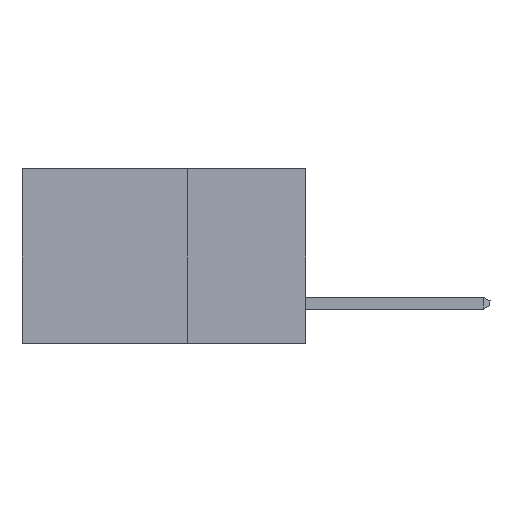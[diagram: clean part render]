
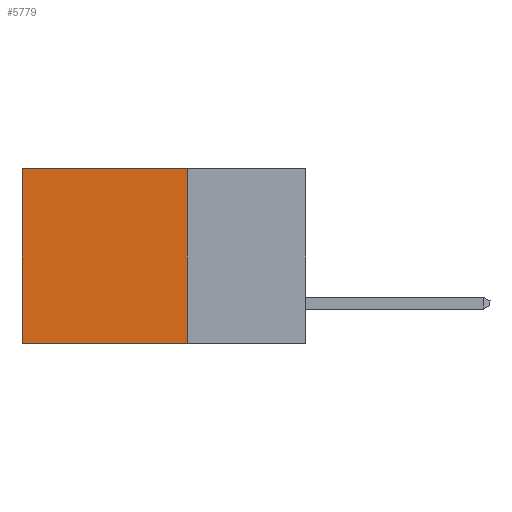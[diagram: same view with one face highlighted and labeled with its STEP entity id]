
A CAD part, left-side view. The second image highlights one B-rep face of the part: STEP entity #5779.
In plain terms, the highlighted planar face has unit normal (-1, 0, 0).
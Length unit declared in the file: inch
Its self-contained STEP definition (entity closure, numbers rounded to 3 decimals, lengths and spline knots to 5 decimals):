
#241 = VERTEX_POINT ( 'NONE', #9505 ) ;
#519 = FACE_OUTER_BOUND ( 'NONE', #14989, .T. ) ;
#837 = CARTESIAN_POINT ( 'NONE',  ( 0.2615, 0.25, -0.37 ) ) ;
#1607 = VECTOR ( 'NONE', #5823, 39.37008 ) ;
#1678 = VERTEX_POINT ( 'NONE', #16621 ) ;
#2047 = CARTESIAN_POINT ( 'NONE',  ( 0.2615, 0.6, 0. ) ) ;
#2447 = LINE ( 'NONE', #19085, #17526 ) ;
#3641 = ORIENTED_EDGE ( 'NONE', *, *, #9684, .F. ) ;
#3858 = CARTESIAN_POINT ( 'NONE',  ( 0.2615, 0.25, -0.37 ) ) ;
#4071 = LINE ( 'NONE', #17266, #1607 ) ;
#5125 = CARTESIAN_POINT ( 'NONE',  ( 0.2615, 0.25, -0.37 ) ) ;
#5719 = DIRECTION ( 'NONE',  ( 0., 0., -1. ) ) ;
#5779 = ADVANCED_FACE ( 'NONE', ( #519 ), #12083, .F. ) ;
#5823 = DIRECTION ( 'NONE',  ( 0., 0., -1. ) ) ;
#5851 = ORIENTED_EDGE ( 'NONE', *, *, #14943, .T. ) ;
#6729 = VECTOR ( 'NONE', #8948, 39.37008 ) ;
#6753 = LINE ( 'NONE', #12467, #20998 ) ;
#8948 = DIRECTION ( 'NONE',  ( 0., 1., 0. ) ) ;
#9505 = CARTESIAN_POINT ( 'NONE',  ( 0.2615, 0.25, 0. ) ) ;
#9684 = EDGE_CURVE ( 'NONE', #13352, #1678, #12294, .T. ) ;
#11070 = EDGE_CURVE ( 'NONE', #17073, #1678, #4071, .T. ) ;
#11278 = DIRECTION ( 'NONE',  ( 0., 1., 0. ) ) ;
#12083 = PLANE ( 'NONE',  #18067 ) ;
#12294 = LINE ( 'NONE', #837, #6729 ) ;
#12467 = CARTESIAN_POINT ( 'NONE',  ( 0.2615, 0.25, -0.37 ) ) ;
#13352 = VERTEX_POINT ( 'NONE', #5125 ) ;
#13461 = EDGE_CURVE ( 'NONE', #241, #13352, #6753, .T. ) ;
#13537 = ORIENTED_EDGE ( 'NONE', *, *, #13461, .F. ) ;
#14943 = EDGE_CURVE ( 'NONE', #241, #17073, #2447, .T. ) ;
#14989 = EDGE_LOOP ( 'NONE', ( #18850, #3641, #13537, #5851 ) ) ;
#16621 = CARTESIAN_POINT ( 'NONE',  ( 0.2615, 0.6, -0.37 ) ) ;
#17049 = DIRECTION ( 'NONE',  ( 1., 0., 0. ) ) ;
#17073 = VERTEX_POINT ( 'NONE', #2047 ) ;
#17266 = CARTESIAN_POINT ( 'NONE',  ( 0.2615, 0.6, -0.37 ) ) ;
#17526 = VECTOR ( 'NONE', #11278, 39.37008 ) ;
#18067 = AXIS2_PLACEMENT_3D ( 'NONE', #3858, #17049, #5719 ) ;
#18850 = ORIENTED_EDGE ( 'NONE', *, *, #11070, .T. ) ;
#19085 = CARTESIAN_POINT ( 'NONE',  ( 0.2615, 0.25, 0. ) ) ;
#20360 = DIRECTION ( 'NONE',  ( 0., 0., -1. ) ) ;
#20998 = VECTOR ( 'NONE', #20360, 39.37008 ) ;
